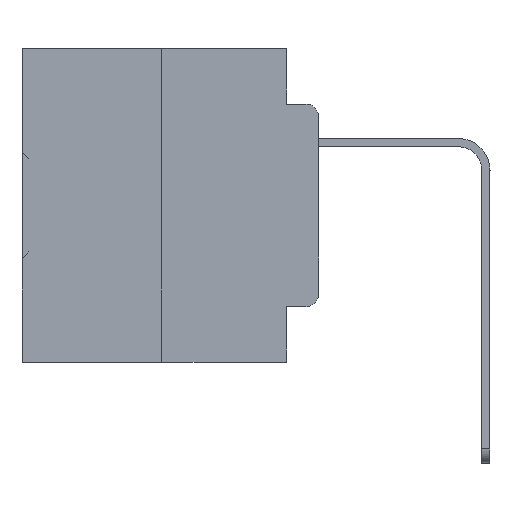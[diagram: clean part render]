
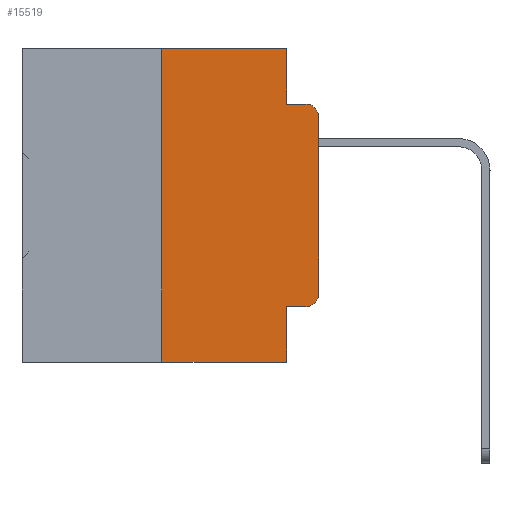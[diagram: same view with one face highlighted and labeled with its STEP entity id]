
A CAD part, left-side view. The second image highlights one B-rep face of the part: STEP entity #15519.
In plain terms, the highlighted planar face has unit normal (-1, 0, 0).
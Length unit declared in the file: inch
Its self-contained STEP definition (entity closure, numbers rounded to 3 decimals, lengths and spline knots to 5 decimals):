
#1070 = EDGE_CURVE ( 'NONE', #24284, #24653, #9793, .T. ) ;
#1236 = EDGE_CURVE ( 'NONE', #24653, #32671, #18280, .T. ) ;
#1389 = EDGE_CURVE ( 'NONE', #2249, #26635, #6184, .T. ) ;
#2249 = VERTEX_POINT ( 'NONE', #6167 ) ;
#2571 = VECTOR ( 'NONE', #33619, 39.37008 ) ;
#2746 = CARTESIAN_POINT ( 'NONE',  ( 0., 0., 0. ) ) ;
#3848 = ORIENTED_EDGE ( 'NONE', *, *, #31298, .F. ) ;
#3864 = ORIENTED_EDGE ( 'NONE', *, *, #7403, .F. ) ;
#4142 = DIRECTION ( 'NONE',  ( 0., -1., 0. ) ) ;
#4401 = CARTESIAN_POINT ( 'NONE',  ( 0., 0.25, 0. ) ) ;
#4458 = EDGE_CURVE ( 'NONE', #10593, #7054, #21866, .T. ) ;
#4611 = VECTOR ( 'NONE', #4142, 39.37008 ) ;
#4726 = VERTEX_POINT ( 'NONE', #12681 ) ;
#6089 = DIRECTION ( 'NONE',  ( 0., 0., -1. ) ) ;
#6167 = CARTESIAN_POINT ( 'NONE',  ( 0., 0., -0.1085 ) ) ;
#6184 = CIRCLE ( 'NONE', #21059, 0.02 ) ;
#6572 = DIRECTION ( 'NONE',  ( 0., -1., 0. ) ) ;
#7054 = VERTEX_POINT ( 'NONE', #10960 ) ;
#7403 = EDGE_CURVE ( 'NONE', #4726, #26635, #32078, .T. ) ;
#7861 = CARTESIAN_POINT ( 'NONE',  ( 0., 0.051, -0.4115 ) ) ;
#8285 = VERTEX_POINT ( 'NONE', #10610 ) ;
#8495 = ORIENTED_EDGE ( 'NONE', *, *, #1236, .T. ) ;
#9235 = CARTESIAN_POINT ( 'NONE',  ( 0., 0.473, 0. ) ) ;
#9793 = LINE ( 'NONE', #7861, #2571 ) ;
#10327 = DIRECTION ( 'NONE',  ( 0., 0., -1. ) ) ;
#10593 = VERTEX_POINT ( 'NONE', #4401 ) ;
#10610 = CARTESIAN_POINT ( 'NONE',  ( 0., 0.051, -0.5 ) ) ;
#10778 = CARTESIAN_POINT ( 'NONE',  ( 0., 0.473, -0.5 ) ) ;
#10960 = CARTESIAN_POINT ( 'NONE',  ( 0., 0.051, 0. ) ) ;
#11052 = DIRECTION ( 'NONE',  ( 0., 0., 1. ) ) ;
#11963 = DIRECTION ( 'NONE',  ( -1., 0., 0. ) ) ;
#12121 = ORIENTED_EDGE ( 'NONE', *, *, #1070, .T. ) ;
#12219 = PLANE ( 'NONE',  #14434 ) ;
#12681 = CARTESIAN_POINT ( 'NONE',  ( 0., 0.051, -0.0885 ) ) ;
#12858 = ORIENTED_EDGE ( 'NONE', *, *, #16907, .F. ) ;
#12887 = ORIENTED_EDGE ( 'NONE', *, *, #14972, .T. ) ;
#12952 = VECTOR ( 'NONE', #15888, 39.37008 ) ;
#13528 = DIRECTION ( 'NONE',  ( 0., -1., 0. ) ) ;
#14434 = AXIS2_PLACEMENT_3D ( 'NONE', #9235, #23772, #32369 ) ;
#14972 = EDGE_CURVE ( 'NONE', #32671, #2249, #16913, .T. ) ;
#14975 = CARTESIAN_POINT ( 'NONE',  ( 0., 0.02, -0.3915 ) ) ;
#15438 = CARTESIAN_POINT ( 'NONE',  ( 0., 0.02, -0.4115 ) ) ;
#15519 = ADVANCED_FACE ( 'NONE', ( #28642 ), #12219, .F. ) ;
#15888 = DIRECTION ( 'NONE',  ( 0., 0., -1. ) ) ;
#15919 = VERTEX_POINT ( 'NONE', #20344 ) ;
#16099 = CARTESIAN_POINT ( 'NONE',  ( 0., 0.25, 0. ) ) ;
#16907 = EDGE_CURVE ( 'NONE', #24284, #8285, #28260, .T. ) ;
#16913 = LINE ( 'NONE', #2746, #29532 ) ;
#16923 = LINE ( 'NONE', #16099, #18721 ) ;
#17819 = VECTOR ( 'NONE', #6089, 39.37008 ) ;
#18280 = CIRCLE ( 'NONE', #19344, 0.02 ) ;
#18710 = EDGE_CURVE ( 'NONE', #7054, #4726, #27265, .T. ) ;
#18721 = VECTOR ( 'NONE', #19211, 39.37008 ) ;
#19211 = DIRECTION ( 'NONE',  ( 0., 0., 1. ) ) ;
#19344 = AXIS2_PLACEMENT_3D ( 'NONE', #14975, #11963, #23261 ) ;
#20344 = CARTESIAN_POINT ( 'NONE',  ( 0., 0.25, -0.5 ) ) ;
#20777 = ORIENTED_EDGE ( 'NONE', *, *, #1389, .T. ) ;
#21056 = VECTOR ( 'NONE', #13528, 39.37008 ) ;
#21059 = AXIS2_PLACEMENT_3D ( 'NONE', #33457, #36015, #10327 ) ;
#21445 = EDGE_LOOP ( 'NONE', ( #12887, #20777, #3864, #30795, #36107, #3848, #26669, #12858, #12121, #8495 ) ) ;
#21866 = LINE ( 'NONE', #32562, #31383 ) ;
#23261 = DIRECTION ( 'NONE',  ( 0., 0., -1. ) ) ;
#23772 = DIRECTION ( 'NONE',  ( 1., 0., 0. ) ) ;
#24284 = VERTEX_POINT ( 'NONE', #34446 ) ;
#24653 = VERTEX_POINT ( 'NONE', #15438 ) ;
#24774 = CARTESIAN_POINT ( 'NONE',  ( 0., 0.051, 0. ) ) ;
#26635 = VERTEX_POINT ( 'NONE', #37255 ) ;
#26669 = ORIENTED_EDGE ( 'NONE', *, *, #29935, .T. ) ;
#26914 = LINE ( 'NONE', #10778, #21056 ) ;
#27265 = LINE ( 'NONE', #28958, #17819 ) ;
#28260 = LINE ( 'NONE', #24774, #12952 ) ;
#28642 = FACE_OUTER_BOUND ( 'NONE', #21445, .T. ) ;
#28958 = CARTESIAN_POINT ( 'NONE',  ( 0., 0.051, 0. ) ) ;
#29532 = VECTOR ( 'NONE', #11052, 39.37008 ) ;
#29935 = EDGE_CURVE ( 'NONE', #15919, #8285, #26914, .T. ) ;
#30795 = ORIENTED_EDGE ( 'NONE', *, *, #18710, .F. ) ;
#30999 = CARTESIAN_POINT ( 'NONE',  ( 0., 0., -0.3915 ) ) ;
#31298 = EDGE_CURVE ( 'NONE', #15919, #10593, #16923, .T. ) ;
#31383 = VECTOR ( 'NONE', #6572, 39.37008 ) ;
#32078 = LINE ( 'NONE', #32442, #4611 ) ;
#32369 = DIRECTION ( 'NONE',  ( 0., 0., -1. ) ) ;
#32442 = CARTESIAN_POINT ( 'NONE',  ( 0., 0.051, -0.0885 ) ) ;
#32562 = CARTESIAN_POINT ( 'NONE',  ( 0., 0.473, 0. ) ) ;
#32671 = VERTEX_POINT ( 'NONE', #30999 ) ;
#33457 = CARTESIAN_POINT ( 'NONE',  ( 0., 0.02, -0.1085 ) ) ;
#33619 = DIRECTION ( 'NONE',  ( 0., -1., 0. ) ) ;
#34446 = CARTESIAN_POINT ( 'NONE',  ( 0., 0.051, -0.4115 ) ) ;
#36015 = DIRECTION ( 'NONE',  ( -1., 0., 0. ) ) ;
#36107 = ORIENTED_EDGE ( 'NONE', *, *, #4458, .F. ) ;
#37255 = CARTESIAN_POINT ( 'NONE',  ( 0., 0.02, -0.0885 ) ) ;
